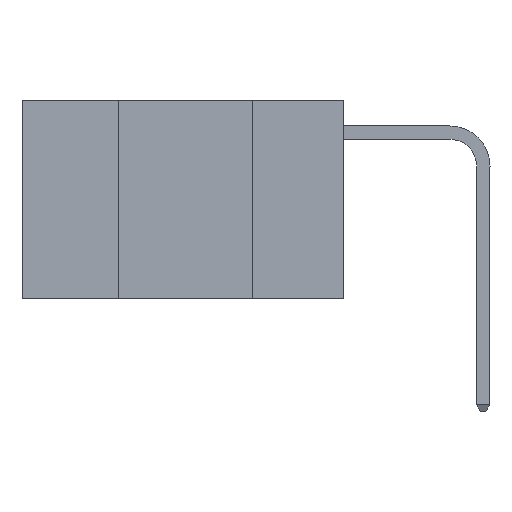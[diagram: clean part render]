
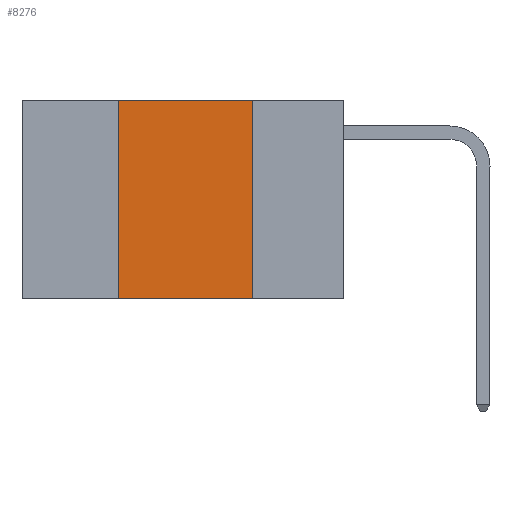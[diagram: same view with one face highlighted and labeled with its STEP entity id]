
A CAD part, left-side view. The second image highlights one B-rep face of the part: STEP entity #8276.
In plain terms, the highlighted planar face has unit normal (-1, 0, 0).
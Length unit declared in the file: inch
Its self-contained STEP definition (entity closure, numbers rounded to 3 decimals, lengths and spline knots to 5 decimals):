
#180 = VERTEX_POINT ( 'NONE', #3366 ) ;
#757 = AXIS2_PLACEMENT_3D ( 'NONE', #1705, #11774, #3164 ) ;
#1420 = EDGE_CURVE ( 'NONE', #2497, #180, #13992, .T. ) ;
#1461 = ORIENTED_EDGE ( 'NONE', *, *, #4434, .F. ) ;
#1705 = CARTESIAN_POINT ( 'NONE',  ( 0., 0.6, 0. ) ) ;
#1731 = VECTOR ( 'NONE', #17334, 39.37008 ) ;
#1789 = CARTESIAN_POINT ( 'NONE',  ( 0., 0.42, 0. ) ) ;
#2497 = VERTEX_POINT ( 'NONE', #13396 ) ;
#2974 = VECTOR ( 'NONE', #16876, 39.37008 ) ;
#3108 = PLANE ( 'NONE',  #757 ) ;
#3164 = DIRECTION ( 'NONE',  ( 0., 0., -1. ) ) ;
#3366 = CARTESIAN_POINT ( 'NONE',  ( 0., 0.17, 0. ) ) ;
#3481 = EDGE_CURVE ( 'NONE', #17791, #15914, #13213, .T. ) ;
#4183 = LINE ( 'NONE', #1789, #12271 ) ;
#4434 = EDGE_CURVE ( 'NONE', #17791, #2497, #4183, .T. ) ;
#4487 = FACE_OUTER_BOUND ( 'NONE', #10849, .T. ) ;
#4560 = ORIENTED_EDGE ( 'NONE', *, *, #5404, .F. ) ;
#5404 = EDGE_CURVE ( 'NONE', #180, #15914, #6618, .T. ) ;
#6141 = DIRECTION ( 'NONE',  ( 0., 0., 1. ) ) ;
#6618 = LINE ( 'NONE', #8176, #7514 ) ;
#7340 = ORIENTED_EDGE ( 'NONE', *, *, #3481, .T. ) ;
#7514 = VECTOR ( 'NONE', #16844, 39.37008 ) ;
#8176 = CARTESIAN_POINT ( 'NONE',  ( 0., 0.17, 0. ) ) ;
#8276 = ADVANCED_FACE ( 'NONE', ( #4487 ), #3108, .F. ) ;
#8349 = CARTESIAN_POINT ( 'NONE',  ( 0., 0.17, -0.37 ) ) ;
#9649 = CARTESIAN_POINT ( 'NONE',  ( 0., 0.6, 0. ) ) ;
#10849 = EDGE_LOOP ( 'NONE', ( #4560, #11430, #1461, #7340 ) ) ;
#11430 = ORIENTED_EDGE ( 'NONE', *, *, #1420, .F. ) ;
#11774 = DIRECTION ( 'NONE',  ( 1., 0., 0. ) ) ;
#12271 = VECTOR ( 'NONE', #6141, 39.37008 ) ;
#13213 = LINE ( 'NONE', #15838, #1731 ) ;
#13396 = CARTESIAN_POINT ( 'NONE',  ( 0., 0.42, 0. ) ) ;
#13992 = LINE ( 'NONE', #9649, #2974 ) ;
#15838 = CARTESIAN_POINT ( 'NONE',  ( 0., 0.6, -0.37 ) ) ;
#15914 = VERTEX_POINT ( 'NONE', #8349 ) ;
#16009 = CARTESIAN_POINT ( 'NONE',  ( 0., 0.42, -0.37 ) ) ;
#16844 = DIRECTION ( 'NONE',  ( 0., 0., -1. ) ) ;
#16876 = DIRECTION ( 'NONE',  ( 0., -1., 0. ) ) ;
#17334 = DIRECTION ( 'NONE',  ( 0., -1., 0. ) ) ;
#17791 = VERTEX_POINT ( 'NONE', #16009 ) ;
